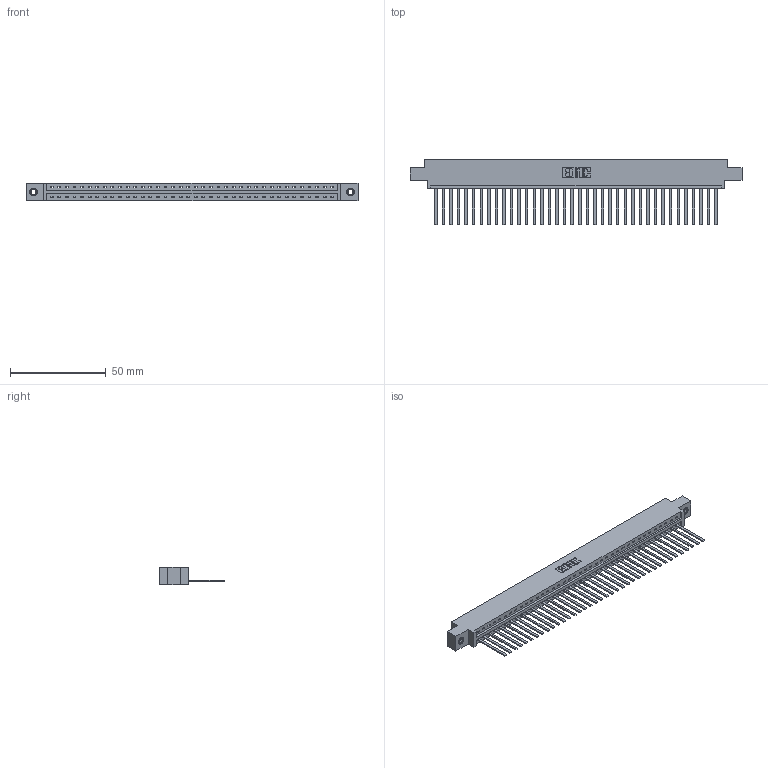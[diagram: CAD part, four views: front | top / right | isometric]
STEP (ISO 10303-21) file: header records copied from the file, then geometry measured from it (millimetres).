
FILE_DESCRIPTION (( 'STEP AP203' ), '1' );
FILE_NAME ('387-038-544-607.STEP', '2019-10-04T16:31:39', ( '' ), ( '' ), 'SwSTEP 2.0', 'SolidWorks 2016', '' );
FILE_SCHEMA (( 'CONFIG_CONTROL_DESIGN' ));
Length unit declared in the file: inch
Products named in the file (4): 345-250-001_345-250-005-103; 337 Part_0.170 Offset - 0.156 Dia-TI; 387-038-544-607; 345-292-001_345-293-144
Assembly tree (41 placements, depth 2):
  387-038-544-607
    337 Part_0.170 Offset - 0.156 Dia-TI
    345-292-001_345-293-144  x38
    345-250-001_345-250-005-103  x2
Bounding box: 173.58 x 34.3 x 9.4 mm (x, y, z)
Volume: 18300.1 mm3; surface area: 20473.4 mm2
Topology: 41 solids, 41 shells, 2306 faces, 6919 edges, 4554 vertices
Faces by surface type: plane 1702, cylinder 588, cone 12, torus 4
Entity records: 29898 total; most frequent: CARTESIAN_POINT 5187, ORIENTED_EDGE 5154, DIRECTION 4403, EDGE_CURVE 2577, VECTOR 2433, LINE 2433, VERTEX_POINT 1712, AXIS2_PLACEMENT_3D 985
